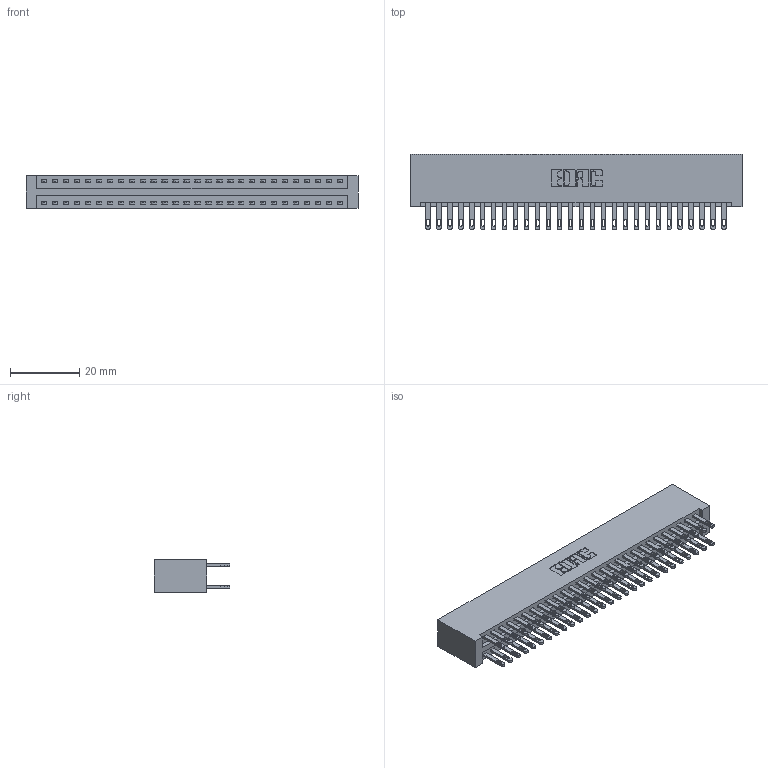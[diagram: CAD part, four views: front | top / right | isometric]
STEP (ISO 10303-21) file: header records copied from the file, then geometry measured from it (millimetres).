
FILE_DESCRIPTION (( 'STEP AP203' ), '1' );
FILE_NAME ('346-056-500-201.STEP', '2018-08-28T02:05:20', ( '' ), ( '' ), 'SwSTEP 2.0', 'SolidWorks 2016', '' );
FILE_SCHEMA (( 'CONFIG_CONTROL_DESIGN' ));
Length unit declared in the file: inch
Products named in the file (3): 346 Part_No Mounting Lugs; 345-292-001_345-293-100; 346-056-500-201
Assembly tree (57 placements, depth 2):
  346-056-500-201
    346 Part_No Mounting Lugs
    345-292-001_345-293-100  x56
Bounding box: 96.14 x 21.84 x 9.4 mm (x, y, z)
Volume: 10010.4 mm3; surface area: 14289.3 mm2
Topology: 57 solids, 57 shells, 2802 faces, 8537 edges, 5690 vertices
Faces by surface type: plane 1696, cylinder 1106
Entity records: 19811 total; most frequent: CARTESIAN_POINT 3280, ORIENTED_EDGE 3214, DIRECTION 2939, EDGE_CURVE 1607, VECTOR 1367, LINE 1367, VERTEX_POINT 1070, AXIS2_PLACEMENT_3D 786
